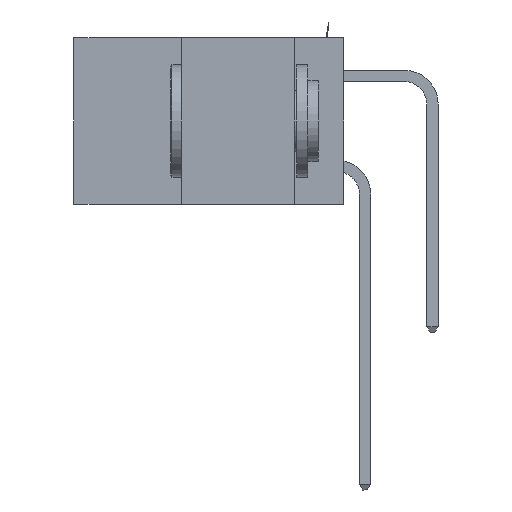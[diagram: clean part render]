
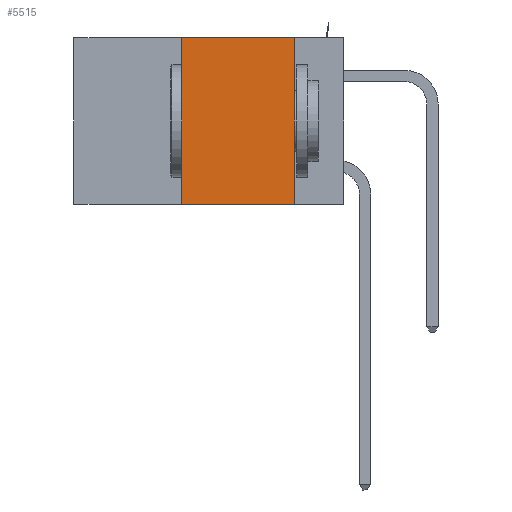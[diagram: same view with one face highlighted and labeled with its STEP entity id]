
A CAD part, left-side view. The second image highlights one B-rep face of the part: STEP entity #5515.
In plain terms, the highlighted planar face has unit normal (-1, 0, 0).
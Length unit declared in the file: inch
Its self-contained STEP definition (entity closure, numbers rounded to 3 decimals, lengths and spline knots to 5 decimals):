
#569 = DIRECTION ( 'NONE',  ( 0., -1., 0. ) ) ;
#1519 = ORIENTED_EDGE ( 'NONE', *, *, #3001, .F. ) ;
#1607 = FACE_OUTER_BOUND ( 'NONE', #8973, .T. ) ;
#2303 = CARTESIAN_POINT ( 'NONE',  ( 0., 0.11, -0.37 ) ) ;
#2665 = CARTESIAN_POINT ( 'NONE',  ( 0., 0.6, 0. ) ) ;
#2765 = DIRECTION ( 'NONE',  ( 0., -1., 0. ) ) ;
#3001 = EDGE_CURVE ( 'NONE', #3283, #13239, #7712, .T. ) ;
#3283 = VERTEX_POINT ( 'NONE', #4391 ) ;
#3732 = EDGE_CURVE ( 'NONE', #10564, #7061, #11242, .T. ) ;
#3755 = PLANE ( 'NONE',  #9213 ) ;
#3776 = CARTESIAN_POINT ( 'NONE',  ( 0., 0.11, 0. ) ) ;
#4311 = ORIENTED_EDGE ( 'NONE', *, *, #7695, .T. ) ;
#4391 = CARTESIAN_POINT ( 'NONE',  ( 0., 0.36, -0.37 ) ) ;
#4498 = DIRECTION ( 'NONE',  ( 0., 0., 1. ) ) ;
#4594 = VECTOR ( 'NONE', #4498, 39.37008 ) ;
#4665 = VECTOR ( 'NONE', #569, 39.37008 ) ;
#5364 = VECTOR ( 'NONE', #11780, 39.37008 ) ;
#5515 = ADVANCED_FACE ( 'NONE', ( #1607 ), #3755, .F. ) ;
#6493 = CARTESIAN_POINT ( 'NONE',  ( 0., 0.6, 0. ) ) ;
#6677 = CARTESIAN_POINT ( 'NONE',  ( 0., 0.36, 0. ) ) ;
#6816 = DIRECTION ( 'NONE',  ( 1., 0., 0. ) ) ;
#6830 = EDGE_CURVE ( 'NONE', #13239, #10564, #7463, .T. ) ;
#6834 = DIRECTION ( 'NONE',  ( 0., 0., -1. ) ) ;
#7061 = VERTEX_POINT ( 'NONE', #2303 ) ;
#7087 = VECTOR ( 'NONE', #2765, 39.37008 ) ;
#7463 = LINE ( 'NONE', #2665, #4665 ) ;
#7695 = EDGE_CURVE ( 'NONE', #3283, #7061, #9613, .T. ) ;
#7712 = LINE ( 'NONE', #6677, #4594 ) ;
#8119 = CARTESIAN_POINT ( 'NONE',  ( 0., 0.36, 0. ) ) ;
#8973 = EDGE_LOOP ( 'NONE', ( #11872, #12170, #1519, #4311 ) ) ;
#9213 = AXIS2_PLACEMENT_3D ( 'NONE', #6493, #6816, #6834 ) ;
#9613 = LINE ( 'NONE', #10083, #7087 ) ;
#10083 = CARTESIAN_POINT ( 'NONE',  ( 0., 0.6, -0.37 ) ) ;
#10564 = VERTEX_POINT ( 'NONE', #3776 ) ;
#11242 = LINE ( 'NONE', #11667, #5364 ) ;
#11667 = CARTESIAN_POINT ( 'NONE',  ( 0., 0.11, 0. ) ) ;
#11780 = DIRECTION ( 'NONE',  ( 0., 0., -1. ) ) ;
#11872 = ORIENTED_EDGE ( 'NONE', *, *, #3732, .F. ) ;
#12170 = ORIENTED_EDGE ( 'NONE', *, *, #6830, .F. ) ;
#13239 = VERTEX_POINT ( 'NONE', #8119 ) ;
